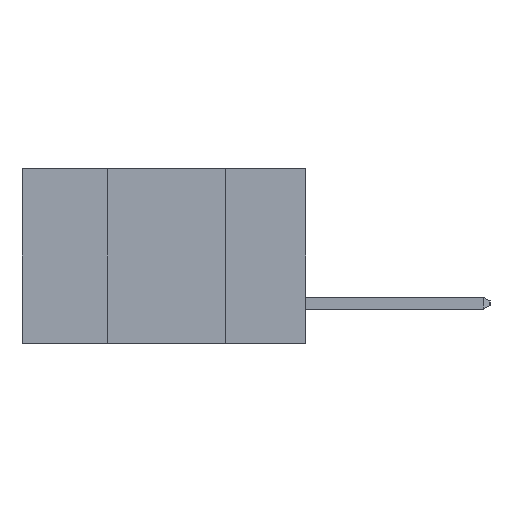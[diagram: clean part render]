
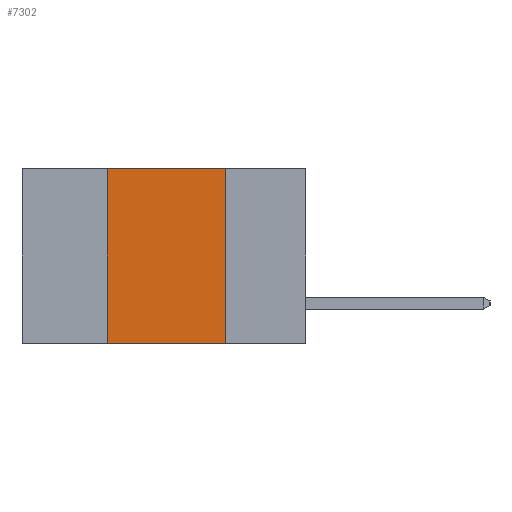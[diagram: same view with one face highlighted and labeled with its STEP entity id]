
A CAD part, left-side view. The second image highlights one B-rep face of the part: STEP entity #7302.
In plain terms, the highlighted planar face has unit normal (-1, 0, 0).
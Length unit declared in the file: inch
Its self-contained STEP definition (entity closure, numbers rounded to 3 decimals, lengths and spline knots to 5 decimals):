
#1021 = LINE ( 'NONE', #11152, #21451 ) ;
#1934 = VERTEX_POINT ( 'NONE', #6172 ) ;
#2352 = VECTOR ( 'NONE', #7531, 39.37008 ) ;
#2426 = EDGE_LOOP ( 'NONE', ( #6315, #11252, #17757, #19851 ) ) ;
#4526 = CARTESIAN_POINT ( 'NONE',  ( 0., 0.6, 0. ) ) ;
#4675 = EDGE_CURVE ( 'NONE', #22996, #1934, #1021, .T. ) ;
#6172 = CARTESIAN_POINT ( 'NONE',  ( 0., 0.17, 0. ) ) ;
#6315 = ORIENTED_EDGE ( 'NONE', *, *, #11536, .F. ) ;
#7302 = ADVANCED_FACE ( 'NONE', ( #14930 ), #22652, .F. ) ;
#7531 = DIRECTION ( 'NONE',  ( 0., 0., 1. ) ) ;
#8313 = LINE ( 'NONE', #15400, #2352 ) ;
#8469 = DIRECTION ( 'NONE',  ( 0., -1., 0. ) ) ;
#8957 = VECTOR ( 'NONE', #12448, 39.37008 ) ;
#9596 = LINE ( 'NONE', #10540, #8957 ) ;
#9949 = VECTOR ( 'NONE', #8469, 39.37008 ) ;
#10540 = CARTESIAN_POINT ( 'NONE',  ( 0., 0.17, -0.37 ) ) ;
#10586 = LINE ( 'NONE', #22191, #9949 ) ;
#11105 = DIRECTION ( 'NONE',  ( 0., -1., 0. ) ) ;
#11112 = VERTEX_POINT ( 'NONE', #13221 ) ;
#11152 = CARTESIAN_POINT ( 'NONE',  ( 0., 0.6, 0. ) ) ;
#11252 = ORIENTED_EDGE ( 'NONE', *, *, #4675, .F. ) ;
#11536 = EDGE_CURVE ( 'NONE', #1934, #21082, #9596, .T. ) ;
#12448 = DIRECTION ( 'NONE',  ( 0., 0., -1. ) ) ;
#13221 = CARTESIAN_POINT ( 'NONE',  ( 0., 0.42, -0.37 ) ) ;
#14930 = FACE_OUTER_BOUND ( 'NONE', #2426, .T. ) ;
#15400 = CARTESIAN_POINT ( 'NONE',  ( 0., 0.42, -0.37 ) ) ;
#15497 = CARTESIAN_POINT ( 'NONE',  ( 0., 0.17, -0.37 ) ) ;
#16204 = AXIS2_PLACEMENT_3D ( 'NONE', #4526, #22478, #22388 ) ;
#16495 = EDGE_CURVE ( 'NONE', #11112, #21082, #10586, .T. ) ;
#17757 = ORIENTED_EDGE ( 'NONE', *, *, #24081, .F. ) ;
#19851 = ORIENTED_EDGE ( 'NONE', *, *, #16495, .T. ) ;
#21082 = VERTEX_POINT ( 'NONE', #15497 ) ;
#21451 = VECTOR ( 'NONE', #11105, 39.37008 ) ;
#22191 = CARTESIAN_POINT ( 'NONE',  ( 0., 0.6, -0.37 ) ) ;
#22388 = DIRECTION ( 'NONE',  ( 0., 0., -1. ) ) ;
#22478 = DIRECTION ( 'NONE',  ( 1., 0., 0. ) ) ;
#22652 = PLANE ( 'NONE',  #16204 ) ;
#22996 = VERTEX_POINT ( 'NONE', #23498 ) ;
#23498 = CARTESIAN_POINT ( 'NONE',  ( 0., 0.42, 0. ) ) ;
#24081 = EDGE_CURVE ( 'NONE', #11112, #22996, #8313, .T. ) ;
